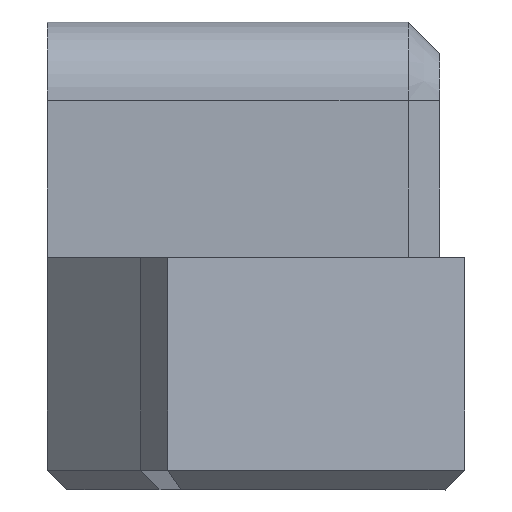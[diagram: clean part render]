
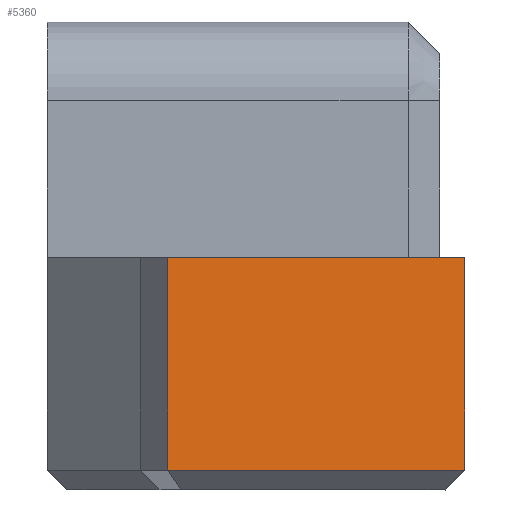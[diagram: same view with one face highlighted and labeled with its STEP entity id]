
A CAD part, left-side view. The second image highlights one B-rep face of the part: STEP entity #5360.
In plain terms, the highlighted planar face has unit normal (-0.73, -0.683, 0).
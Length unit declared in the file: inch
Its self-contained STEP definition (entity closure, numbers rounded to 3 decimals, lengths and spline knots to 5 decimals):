
#1 = LINE ( 'NONE', #349, #4306 ) ;
#119 = VECTOR ( 'NONE', #4534, 39.37008 ) ;
#120 = VERTEX_POINT ( 'NONE', #3822 ) ;
#289 = DIRECTION ( 'NONE',  ( 0.684, -0.73, 0. ) ) ;
#349 = CARTESIAN_POINT ( 'NONE',  ( -4.47442, 1.148, 1.09346 ) ) ;
#382 = DIRECTION ( 'NONE',  ( 0., 0., 1. ) ) ;
#778 = EDGE_CURVE ( 'NONE', #2292, #4454, #4537, .T. ) ;
#1317 = CARTESIAN_POINT ( 'NONE',  ( -4.91753, 1.6212, 2.40297 ) ) ;
#1370 = VECTOR ( 'NONE', #2886, 39.37008 ) ;
#1541 = ORIENTED_EDGE ( 'NONE', *, *, #5166, .T. ) ;
#1824 = PLANE ( 'NONE',  #4975 ) ;
#2292 = VERTEX_POINT ( 'NONE', #1317 ) ;
#2487 = LINE ( 'NONE', #3292, #119 ) ;
#2540 = FACE_OUTER_BOUND ( 'NONE', #2542, .T. ) ;
#2542 = EDGE_LOOP ( 'NONE', ( #3671, #5366, #1541, #4680 ) ) ;
#2580 = CARTESIAN_POINT ( 'NONE',  ( -4.91753, 1.6212, 2.74197 ) ) ;
#2667 = CARTESIAN_POINT ( 'NONE',  ( -4.47442, 1.148, 2.40297 ) ) ;
#2886 = DIRECTION ( 'NONE',  ( 0.684, -0.73, 0. ) ) ;
#3108 = CARTESIAN_POINT ( 'NONE',  ( -4.91753, 1.6212, 4.05299 ) ) ;
#3150 = VERTEX_POINT ( 'NONE', #2667 ) ;
#3292 = CARTESIAN_POINT ( 'NONE',  ( -4.47442, 1.148, 2.40297 ) ) ;
#3402 = LINE ( 'NONE', #3647, #1370 ) ;
#3647 = CARTESIAN_POINT ( 'NONE',  ( -4.47442, 1.148, 2.74197 ) ) ;
#3671 = ORIENTED_EDGE ( 'NONE', *, *, #778, .F. ) ;
#3822 = CARTESIAN_POINT ( 'NONE',  ( -4.47442, 1.148, 2.74197 ) ) ;
#3829 = VECTOR ( 'NONE', #4324, 39.37008 ) ;
#4129 = CARTESIAN_POINT ( 'NONE',  ( -4.92154, 1.62549, 4.05299 ) ) ;
#4306 = VECTOR ( 'NONE', #382, 39.37008 ) ;
#4324 = DIRECTION ( 'NONE',  ( 0., 0., 1. ) ) ;
#4454 = VERTEX_POINT ( 'NONE', #2580 ) ;
#4530 = DIRECTION ( 'NONE',  ( -0.73, -0.684, 0. ) ) ;
#4534 = DIRECTION ( 'NONE',  ( 0.684, -0.73, 0. ) ) ;
#4537 = LINE ( 'NONE', #3108, #3829 ) ;
#4646 = EDGE_CURVE ( 'NONE', #4454, #120, #3402, .T. ) ;
#4680 = ORIENTED_EDGE ( 'NONE', *, *, #4646, .F. ) ;
#4975 = AXIS2_PLACEMENT_3D ( 'NONE', #4129, #4530, #289 ) ;
#5062 = EDGE_CURVE ( 'NONE', #2292, #3150, #2487, .T. ) ;
#5166 = EDGE_CURVE ( 'NONE', #3150, #120, #1, .T. ) ;
#5360 = ADVANCED_FACE ( 'NONE', ( #2540 ), #1824, .T. ) ;
#5366 = ORIENTED_EDGE ( 'NONE', *, *, #5062, .T. ) ;
